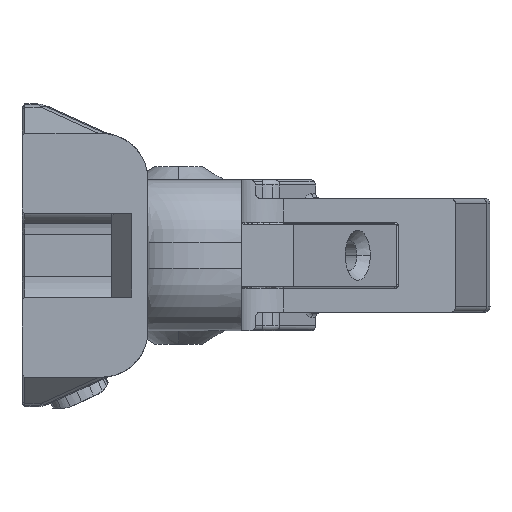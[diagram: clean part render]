
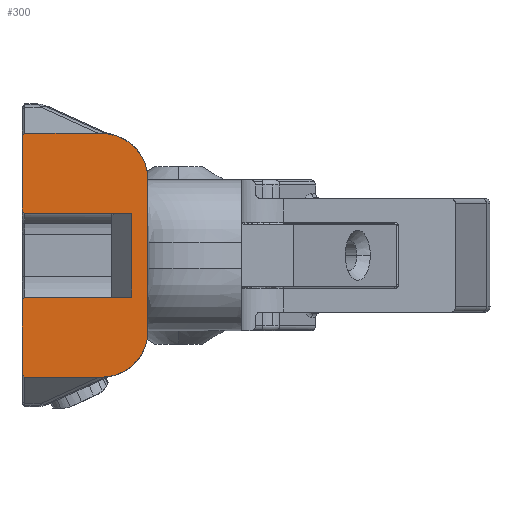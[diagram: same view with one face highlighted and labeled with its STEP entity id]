
A CAD part, left-side view. The second image highlights one B-rep face of the part: STEP entity #300.
In plain terms, the highlighted planar face has unit normal (-1, 0, 0).
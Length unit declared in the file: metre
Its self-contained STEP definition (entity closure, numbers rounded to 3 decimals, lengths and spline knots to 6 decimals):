
#300=ADVANCED_FACE('4:394',(#1224),#1225,.F.);
#1224=FACE_OUTER_BOUND('',#2610,.T.);
#1225=PLANE('',#2611);
#2610=EDGE_LOOP('',(#7477,#7478,#7479,#7480,#7481,#7482,#7483,#7484,#7485,#7486,#7487,#7488,#7489,#7490));
#2611=AXIS2_PLACEMENT_3D('',#7491,#7492,#7493);
#7477=ORIENTED_EDGE('',*,*,#11659,.T.);
#7478=ORIENTED_EDGE('',*,*,#11660,.T.);
#7479=ORIENTED_EDGE('',*,*,#11661,.T.);
#7480=ORIENTED_EDGE('',*,*,#11662,.T.);
#7481=ORIENTED_EDGE('',*,*,#11663,.T.);
#7482=ORIENTED_EDGE('',*,*,#11664,.T.);
#7483=ORIENTED_EDGE('',*,*,#11665,.T.);
#7484=ORIENTED_EDGE('',*,*,#11666,.T.);
#7485=ORIENTED_EDGE('',*,*,#11667,.T.);
#7486=ORIENTED_EDGE('',*,*,#11668,.T.);
#7487=ORIENTED_EDGE('',*,*,#11669,.T.);
#7488=ORIENTED_EDGE('',*,*,#11670,.T.);
#7489=ORIENTED_EDGE('',*,*,#11671,.T.);
#7490=ORIENTED_EDGE('',*,*,#11672,.T.);
#7491=CARTESIAN_POINT('',(-0.193511,0.005963,-0.025461));
#7492=DIRECTION('',(1.,0.,0.));
#7493=DIRECTION('',(0.,-0.024,-1.));
#11659=EDGE_CURVE('4:3019',#14091,#14092,#14093,.T.);
#11660=EDGE_CURVE('4:3022',#14092,#14094,#14095,.T.);
#11661=EDGE_CURVE('4:3025',#14094,#14096,#14097,.T.);
#11662=EDGE_CURVE('4:3028',#14096,#14098,#14099,.T.);
#11663=EDGE_CURVE('4:3031',#14098,#14100,#14101,.T.);
#11664=EDGE_CURVE('4:3034',#14100,#14102,#14103,.T.);
#11665=EDGE_CURVE('4:3037',#14102,#14104,#14105,.T.);
#11666=EDGE_CURVE('4:3040',#14104,#14106,#14107,.T.);
#11667=EDGE_CURVE('4:3043',#14106,#14108,#14109,.T.);
#11668=EDGE_CURVE('4:3046',#14108,#14110,#14111,.T.);
#11669=EDGE_CURVE('4:3049',#14110,#14112,#14113,.T.);
#11670=EDGE_CURVE('4:3052',#14112,#14114,#14115,.T.);
#11671=EDGE_CURVE('4:3055',#14114,#14116,#14117,.T.);
#11672=EDGE_CURVE('4:3058',#14116,#14091,#14118,.T.);
#14091=VERTEX_POINT('',#18925);
#14092=VERTEX_POINT('',#18926);
#14093=LINE('',#18927,#18928);
#14094=VERTEX_POINT('',#18929);
#14095=LINE('',#18930,#18931);
#14096=VERTEX_POINT('',#18932);
#14097=LINE('',#18933,#18934);
#14098=VERTEX_POINT('',#18935);
#14099=LINE('',#18936,#18937);
#14100=VERTEX_POINT('',#18938);
#14101=LINE('',#18939,#18940);
#14102=VERTEX_POINT('',#18941);
#14103=LINE('',#18942,#18943);
#14104=VERTEX_POINT('',#18944);
#14105=LINE('',#18945,#18946);
#14106=VERTEX_POINT('',#18947);
#14107=CIRCLE('',#18948,0.007057);
#14108=VERTEX_POINT('',#18949);
#14109=LINE('',#18950,#18951);
#14110=VERTEX_POINT('',#18952);
#14111=CIRCLE('',#18953,0.007057);
#14112=VERTEX_POINT('',#18954);
#14113=LINE('',#18955,#18956);
#14114=VERTEX_POINT('',#18957);
#14115=LINE('',#18958,#18959);
#14116=VERTEX_POINT('',#18960);
#14117=LINE('',#18961,#18962);
#14118=LINE('',#18963,#18964);
#18925=CARTESIAN_POINT('',(-0.193512,0.005241,0.00735));
#18926=CARTESIAN_POINT('',(-0.193515,-0.011059,0.00735));
#18927=CARTESIAN_POINT('',(-0.193512,0.001527,0.00735));
#18928=VECTOR('',#27293,1.0);
#18929=CARTESIAN_POINT('',(-0.193515,-0.011059,-0.00535));
#18930=CARTESIAN_POINT('',(-0.193515,-0.011059,-0.01223));
#18931=VECTOR('',#27294,1.0);
#18932=CARTESIAN_POINT('',(-0.193511,0.005241,-0.00535));
#18933=CARTESIAN_POINT('',(-0.193512,0.001527,-0.00535));
#18934=VECTOR('',#27295,1.0);
#18935=CARTESIAN_POINT('',(-0.193511,0.005641,-0.00575));
#18936=CARTESIAN_POINT('',(-0.19351,0.010549,-0.010658));
#18937=VECTOR('',#27296,1.0);
#18938=CARTESIAN_POINT('',(-0.193511,0.005641,-0.017167));
#18939=CARTESIAN_POINT('',(-0.193511,0.005641,-0.018459));
#18940=VECTOR('',#27297,1.0);
#18941=CARTESIAN_POINT('',(-0.193511,0.005241,-0.017567));
#18942=CARTESIAN_POINT('',(-0.193512,0.003548,-0.01926));
#18943=VECTOR('',#27298,1.0);
#18944=CARTESIAN_POINT('',(-0.193514,-0.006479,-0.017567));
#18945=CARTESIAN_POINT('',(-0.193512,0.002672,-0.017567));
#18946=VECTOR('',#27299,1.0);
#18947=CARTESIAN_POINT('',(-0.193515,-0.013536,-0.010509));
#18948=AXIS2_PLACEMENT_3D('',#27300,#27301,#27302);
#18949=CARTESIAN_POINT('',(-0.193515,-0.013536,0.012509));
#18950=CARTESIAN_POINT('',(-0.193515,-0.013536,-0.01223));
#18951=VECTOR('',#27303,1.0);
#18952=CARTESIAN_POINT('',(-0.193514,-0.006479,0.019567));
#18953=AXIS2_PLACEMENT_3D('',#27304,#27305,#27306);
#18954=CARTESIAN_POINT('',(-0.193512,0.005241,0.019567));
#18955=CARTESIAN_POINT('',(-0.193512,0.002672,0.019567));
#18956=VECTOR('',#27307,1.0);
#18957=CARTESIAN_POINT('',(-0.193512,0.005641,0.019167));
#18958=CARTESIAN_POINT('',(-0.193509,0.016778,0.008029));
#18959=VECTOR('',#27308,1.0);
#18960=CARTESIAN_POINT('',(-0.193511,0.005641,0.00775));
#18961=CARTESIAN_POINT('',(-0.193511,0.005641,-0.006001));
#18962=VECTOR('',#27309,1.0);
#18963=CARTESIAN_POINT('',(-0.193513,-0.002681,-0.000572));
#18964=VECTOR('',#27310,1.0);
#27293=DIRECTION('',(0.,-1.,0.));
#27294=DIRECTION('',(0.,0.,-1.));
#27295=DIRECTION('',(0.,1.,0.));
#27296=DIRECTION('',(0.,0.707,-0.707));
#27297=DIRECTION('',(0.,0.,-1.));
#27298=DIRECTION('',(0.,-0.707,-0.707));
#27299=DIRECTION('',(0.,-1.,0.));
#27300=CARTESIAN_POINT('',(-0.193514,-0.006479,-0.010509));
#27301=DIRECTION('',(-1.,0.,0.));
#27302=DIRECTION('',(0.,-1.,0.024));
#27303=DIRECTION('',(0.,0.,1.));
#27304=CARTESIAN_POINT('',(-0.193514,-0.006479,0.012509));
#27305=DIRECTION('',(-1.,0.,0.));
#27306=DIRECTION('',(0.,-1.,0.024));
#27307=DIRECTION('',(0.,1.,0.));
#27308=DIRECTION('',(0.,0.707,-0.707));
#27309=DIRECTION('',(0.,0.,-1.));
#27310=DIRECTION('',(0.,-0.707,-0.707));
